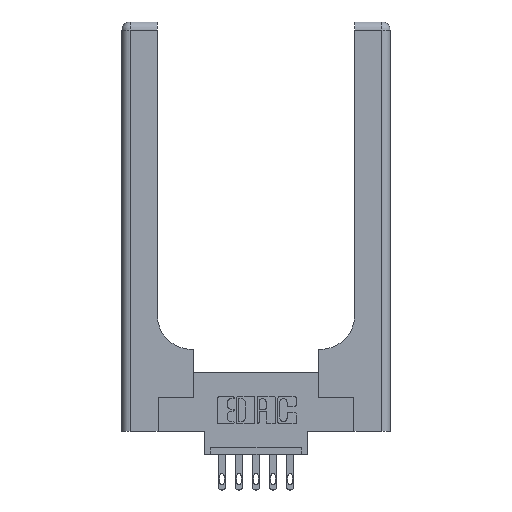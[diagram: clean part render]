
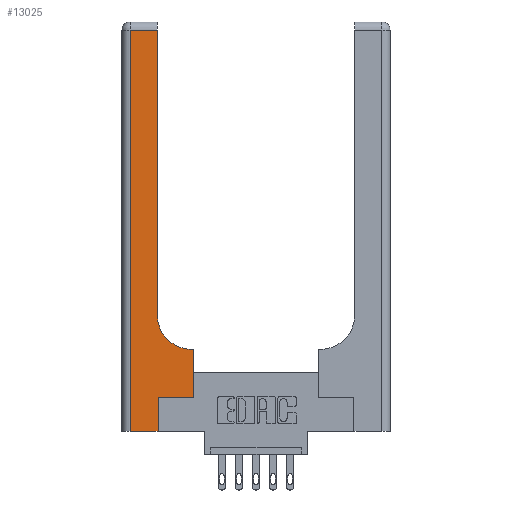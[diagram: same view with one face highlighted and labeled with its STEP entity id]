
A CAD part, top view. The second image highlights one B-rep face of the part: STEP entity #13025.
In plain terms, the highlighted planar face has unit normal (0, 0, 1).
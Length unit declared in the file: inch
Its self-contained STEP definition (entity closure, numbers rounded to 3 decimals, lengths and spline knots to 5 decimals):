
#88 = AXIS2_PLACEMENT_3D ( 'NONE', #4450, #8512, #12762 ) ;
#308 = ORIENTED_EDGE ( 'NONE', *, *, #10587, .T. ) ;
#318 = VERTEX_POINT ( 'NONE', #11399 ) ;
#521 = CIRCLE ( 'NONE', #88, 0.25 ) ;
#704 = LINE ( 'NONE', #13446, #3341 ) ;
#1014 = VERTEX_POINT ( 'NONE', #4839 ) ;
#1330 = VECTOR ( 'NONE', #1379, 39.37008 ) ;
#1379 = DIRECTION ( 'NONE',  ( 0., -1., 0. ) ) ;
#1402 = VERTEX_POINT ( 'NONE', #1424 ) ;
#1424 = CARTESIAN_POINT ( 'NONE',  ( 0.265, 0., 0.37 ) ) ;
#1502 = VERTEX_POINT ( 'NONE', #5030 ) ;
#1749 = LINE ( 'NONE', #13379, #3043 ) ;
#1764 = VECTOR ( 'NONE', #9551, 39.37008 ) ;
#2128 = ORIENTED_EDGE ( 'NONE', *, *, #10337, .T. ) ;
#2714 = PLANE ( 'NONE',  #8861 ) ;
#2858 = DIRECTION ( 'NONE',  ( 1., 0., 0. ) ) ;
#2937 = ORIENTED_EDGE ( 'NONE', *, *, #7433, .T. ) ;
#3043 = VECTOR ( 'NONE', #3830, 39.37008 ) ;
#3082 = EDGE_CURVE ( 'NONE', #318, #11997, #11577, .T. ) ;
#3305 = VERTEX_POINT ( 'NONE', #3615 ) ;
#3341 = VECTOR ( 'NONE', #2858, 39.37008 ) ;
#3615 = CARTESIAN_POINT ( 'NONE',  ( 0.265, 0.25, 0.37 ) ) ;
#3775 = EDGE_CURVE ( 'NONE', #4309, #1502, #5899, .T. ) ;
#3809 = ORIENTED_EDGE ( 'NONE', *, *, #3082, .T. ) ;
#3830 = DIRECTION ( 'NONE',  ( -1., 0., 0. ) ) ;
#4022 = VECTOR ( 'NONE', #4146, 39.37008 ) ;
#4146 = DIRECTION ( 'NONE',  ( 0., 1., 0. ) ) ;
#4246 = ORIENTED_EDGE ( 'NONE', *, *, #11303, .T. ) ;
#4309 = VERTEX_POINT ( 'NONE', #10532 ) ;
#4442 = EDGE_CURVE ( 'NONE', #10544, #318, #521, .T. ) ;
#4450 = CARTESIAN_POINT ( 'NONE',  ( 0.51, 0.85, 0.37 ) ) ;
#4639 = CARTESIAN_POINT ( 'NONE',  ( 0.51, 0.6, 0.37 ) ) ;
#4772 = CARTESIAN_POINT ( 'NONE',  ( 0.06, 3., 0.37 ) ) ;
#4832 = VECTOR ( 'NONE', #7150, 39.37008 ) ;
#4839 = CARTESIAN_POINT ( 'NONE',  ( 0.528, 0.6, 0.37 ) ) ;
#5030 = CARTESIAN_POINT ( 'NONE',  ( 0.06, 0., 0.37 ) ) ;
#5088 = DIRECTION ( 'NONE',  ( 0., 1., 0. ) ) ;
#5290 = LINE ( 'NONE', #10786, #1764 ) ;
#5899 = LINE ( 'NONE', #4772, #1330 ) ;
#5981 = DIRECTION ( 'NONE',  ( -1., 0., 0. ) ) ;
#6214 = CARTESIAN_POINT ( 'NONE',  ( 0.528, 0.25, 0.37 ) ) ;
#6287 = EDGE_CURVE ( 'NONE', #11997, #4309, #12367, .T. ) ;
#6782 = ORIENTED_EDGE ( 'NONE', *, *, #7723, .T. ) ;
#7025 = CARTESIAN_POINT ( 'NONE',  ( 0., 3., 0.37 ) ) ;
#7117 = CARTESIAN_POINT ( 'NONE',  ( 0.26, 3., 0.37 ) ) ;
#7150 = DIRECTION ( 'NONE',  ( -1., 0., 0. ) ) ;
#7305 = ORIENTED_EDGE ( 'NONE', *, *, #6287, .T. ) ;
#7433 = EDGE_CURVE ( 'NONE', #3305, #11005, #5290, .T. ) ;
#7446 = CARTESIAN_POINT ( 'NONE',  ( 0.26, 2.94, 0.37 ) ) ;
#7489 = CARTESIAN_POINT ( 'NONE',  ( 0.528, 0.25, 0.37 ) ) ;
#7676 = EDGE_LOOP ( 'NONE', ( #3809, #7305, #10761, #2128, #6782, #2937, #308, #4246, #9605 ) ) ;
#7723 = EDGE_CURVE ( 'NONE', #1402, #3305, #13694, .T. ) ;
#8191 = VECTOR ( 'NONE', #5088, 39.37008 ) ;
#8512 = DIRECTION ( 'NONE',  ( 0., 0., -1. ) ) ;
#8861 = AXIS2_PLACEMENT_3D ( 'NONE', #7025, #13292, #5981 ) ;
#9377 = DIRECTION ( 'NONE',  ( 0., 1., 0. ) ) ;
#9551 = DIRECTION ( 'NONE',  ( 1., 0., 0. ) ) ;
#9605 = ORIENTED_EDGE ( 'NONE', *, *, #4442, .T. ) ;
#10337 = EDGE_CURVE ( 'NONE', #1502, #1402, #704, .T. ) ;
#10532 = CARTESIAN_POINT ( 'NONE',  ( 0.06, 2.94, 0.37 ) ) ;
#10544 = VERTEX_POINT ( 'NONE', #4639 ) ;
#10563 = CARTESIAN_POINT ( 'NONE',  ( 0.265, 0., 0.37 ) ) ;
#10587 = EDGE_CURVE ( 'NONE', #11005, #1014, #13624, .T. ) ;
#10761 = ORIENTED_EDGE ( 'NONE', *, *, #3775, .T. ) ;
#10786 = CARTESIAN_POINT ( 'NONE',  ( 0.265, 0.25, 0.37 ) ) ;
#11005 = VERTEX_POINT ( 'NONE', #6214 ) ;
#11187 = CARTESIAN_POINT ( 'NONE',  ( 0., 2.94, 0.37 ) ) ;
#11206 = FACE_OUTER_BOUND ( 'NONE', #7676, .T. ) ;
#11303 = EDGE_CURVE ( 'NONE', #1014, #10544, #1749, .T. ) ;
#11399 = CARTESIAN_POINT ( 'NONE',  ( 0.26, 0.85, 0.37 ) ) ;
#11577 = LINE ( 'NONE', #7117, #8191 ) ;
#11599 = VECTOR ( 'NONE', #9377, 39.37008 ) ;
#11997 = VERTEX_POINT ( 'NONE', #7446 ) ;
#12367 = LINE ( 'NONE', #11187, #4832 ) ;
#12762 = DIRECTION ( 'NONE',  ( 1., 0., 0. ) ) ;
#13025 = ADVANCED_FACE ( 'NONE', ( #11206 ), #2714, .F. ) ;
#13292 = DIRECTION ( 'NONE',  ( 0., 0., -1. ) ) ;
#13379 = CARTESIAN_POINT ( 'NONE',  ( 0.26, 0.6, 0.37 ) ) ;
#13446 = CARTESIAN_POINT ( 'NONE',  ( 0., 0., 0.37 ) ) ;
#13624 = LINE ( 'NONE', #7489, #11599 ) ;
#13694 = LINE ( 'NONE', #10563, #4022 ) ;
